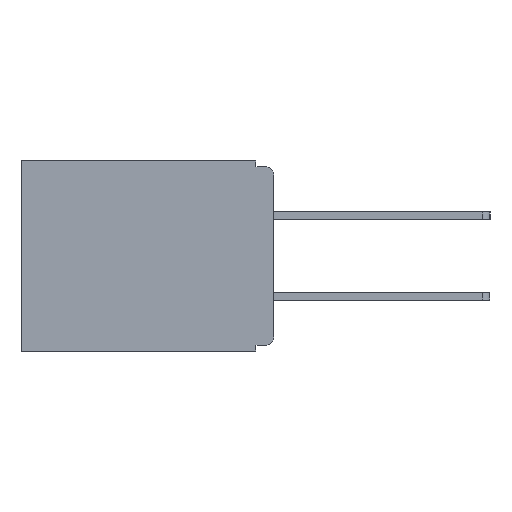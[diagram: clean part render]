
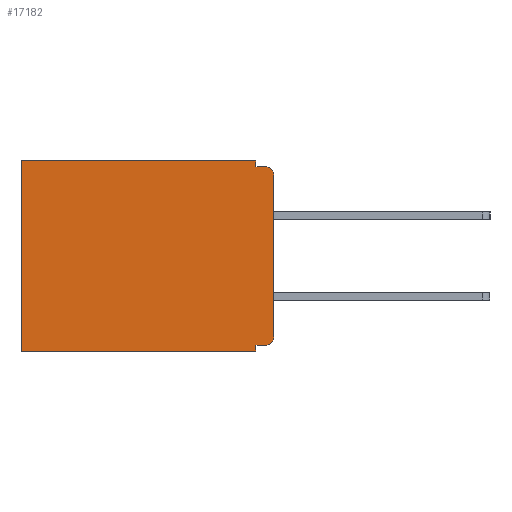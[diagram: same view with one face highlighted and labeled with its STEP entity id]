
A CAD part, left-side view. The second image highlights one B-rep face of the part: STEP entity #17182.
In plain terms, the highlighted planar face has unit normal (-1, 0, 0).
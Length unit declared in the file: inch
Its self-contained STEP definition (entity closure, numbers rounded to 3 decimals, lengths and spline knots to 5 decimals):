
#286 = DIRECTION ( 'NONE',  ( 0., 0., -1. ) ) ;
#375 = ORIENTED_EDGE ( 'NONE', *, *, #14179, .F. ) ;
#651 = LINE ( 'NONE', #19737, #20447 ) ;
#837 = EDGE_CURVE ( 'NONE', #881, #17646, #8882, .T. ) ;
#881 = VERTEX_POINT ( 'NONE', #23216 ) ;
#1035 = LINE ( 'NONE', #2843, #15155 ) ;
#1166 = ORIENTED_EDGE ( 'NONE', *, *, #12074, .T. ) ;
#1326 = VERTEX_POINT ( 'NONE', #3470 ) ;
#2004 = AXIS2_PLACEMENT_3D ( 'NONE', #9203, #22549, #11126 ) ;
#2218 = ORIENTED_EDGE ( 'NONE', *, *, #837, .F. ) ;
#2843 = CARTESIAN_POINT ( 'NONE',  ( 0.3, 0., -0.01 ) ) ;
#3128 = CARTESIAN_POINT ( 'NONE',  ( 0.3, 0.031, 0. ) ) ;
#3470 = CARTESIAN_POINT ( 'NONE',  ( 0.3, 0.031, 0. ) ) ;
#3496 = DIRECTION ( 'NONE',  ( 0., 1., 0. ) ) ;
#5076 = DIRECTION ( 'NONE',  ( 0., 0., -1. ) ) ;
#5280 = CARTESIAN_POINT ( 'NONE',  ( 0.3, 0.015, -0.01 ) ) ;
#5361 = DIRECTION ( 'NONE',  ( 1., 0., 0. ) ) ;
#5703 = EDGE_CURVE ( 'NONE', #19133, #17646, #16681, .T. ) ;
#5920 = VERTEX_POINT ( 'NONE', #5280 ) ;
#6975 = VERTEX_POINT ( 'NONE', #13153 ) ;
#7136 = EDGE_LOOP ( 'NONE', ( #2218, #1166, #375, #15048, #14699, #13847, #13239, #12984, #12619, #12115 ) ) ;
#7376 = VERTEX_POINT ( 'NONE', #16250 ) ;
#8443 = CARTESIAN_POINT ( 'NONE',  ( 0.3, 0.437, 0. ) ) ;
#8515 = DIRECTION ( 'NONE',  ( 0., -1., 0. ) ) ;
#8859 = CARTESIAN_POINT ( 'NONE',  ( 0.3, 0.031, -0.33 ) ) ;
#8880 = LINE ( 'NONE', #8859, #22339 ) ;
#8882 = LINE ( 'NONE', #13978, #19072 ) ;
#9203 = CARTESIAN_POINT ( 'NONE',  ( 0.3, 0.015, -0.025 ) ) ;
#9400 = CARTESIAN_POINT ( 'NONE',  ( 0.3, 0.437, -0.33 ) ) ;
#9470 = AXIS2_PLACEMENT_3D ( 'NONE', #19994, #11107, #286 ) ;
#9677 = EDGE_CURVE ( 'NONE', #13610, #7376, #20761, .T. ) ;
#9882 = CARTESIAN_POINT ( 'NONE',  ( 0.3, 0., -0.32 ) ) ;
#10412 = VECTOR ( 'NONE', #5076, 39.37008 ) ;
#10506 = EDGE_CURVE ( 'NONE', #10758, #7376, #651, .T. ) ;
#10758 = VERTEX_POINT ( 'NONE', #12755 ) ;
#11087 = CARTESIAN_POINT ( 'NONE',  ( 0.3, 0., 0. ) ) ;
#11107 = DIRECTION ( 'NONE',  ( -1., 0., 0. ) ) ;
#11126 = DIRECTION ( 'NONE',  ( 0., 0., -1. ) ) ;
#11375 = FACE_OUTER_BOUND ( 'NONE', #7136, .T. ) ;
#11613 = CARTESIAN_POINT ( 'NONE',  ( 0.3, 0.031, -0.01 ) ) ;
#12074 = EDGE_CURVE ( 'NONE', #881, #5920, #12242, .T. ) ;
#12115 = ORIENTED_EDGE ( 'NONE', *, *, #5703, .T. ) ;
#12242 = CIRCLE ( 'NONE', #2004, 0.015 ) ;
#12579 = VECTOR ( 'NONE', #3496, 39.37008 ) ;
#12619 = ORIENTED_EDGE ( 'NONE', *, *, #22333, .F. ) ;
#12755 = CARTESIAN_POINT ( 'NONE',  ( 0.3, 0.031, -0.33 ) ) ;
#12984 = ORIENTED_EDGE ( 'NONE', *, *, #18687, .F. ) ;
#13153 = CARTESIAN_POINT ( 'NONE',  ( 0.3, 0.031, -0.32 ) ) ;
#13239 = ORIENTED_EDGE ( 'NONE', *, *, #10506, .F. ) ;
#13610 = VERTEX_POINT ( 'NONE', #8443 ) ;
#13847 = ORIENTED_EDGE ( 'NONE', *, *, #9677, .T. ) ;
#13978 = CARTESIAN_POINT ( 'NONE',  ( 0.3, 0., -0.33 ) ) ;
#14087 = VECTOR ( 'NONE', #21343, 39.37008 ) ;
#14179 = EDGE_CURVE ( 'NONE', #22879, #5920, #1035, .T. ) ;
#14683 = LINE ( 'NONE', #9882, #14087 ) ;
#14699 = ORIENTED_EDGE ( 'NONE', *, *, #21457, .T. ) ;
#14764 = CARTESIAN_POINT ( 'NONE',  ( 0.3, 0., -0.305 ) ) ;
#15048 = ORIENTED_EDGE ( 'NONE', *, *, #23754, .F. ) ;
#15078 = VECTOR ( 'NONE', #24606, 39.37008 ) ;
#15155 = VECTOR ( 'NONE', #8515, 39.37008 ) ;
#15517 = LINE ( 'NONE', #3128, #10412 ) ;
#16250 = CARTESIAN_POINT ( 'NONE',  ( 0.3, 0.437, -0.33 ) ) ;
#16681 = CIRCLE ( 'NONE', #9470, 0.015 ) ;
#16805 = CARTESIAN_POINT ( 'NONE',  ( 0.3, 0., -0.33 ) ) ;
#17182 = ADVANCED_FACE ( 'NONE', ( #11375 ), #20560, .F. ) ;
#17646 = VERTEX_POINT ( 'NONE', #14764 ) ;
#17699 = LINE ( 'NONE', #11087, #12579 ) ;
#18687 = EDGE_CURVE ( 'NONE', #6975, #10758, #8880, .T. ) ;
#18713 = DIRECTION ( 'NONE',  ( 0., 0., -1. ) ) ;
#18759 = AXIS2_PLACEMENT_3D ( 'NONE', #16805, #5361, #18713 ) ;
#19072 = VECTOR ( 'NONE', #19273, 39.37008 ) ;
#19133 = VERTEX_POINT ( 'NONE', #23594 ) ;
#19273 = DIRECTION ( 'NONE',  ( 0., 0., -1. ) ) ;
#19737 = CARTESIAN_POINT ( 'NONE',  ( 0.3, 0., -0.33 ) ) ;
#19994 = CARTESIAN_POINT ( 'NONE',  ( 0.3, 0.015, -0.305 ) ) ;
#20447 = VECTOR ( 'NONE', #23528, 39.37008 ) ;
#20560 = PLANE ( 'NONE',  #18759 ) ;
#20761 = LINE ( 'NONE', #9400, #15078 ) ;
#21343 = DIRECTION ( 'NONE',  ( 0., 1., 0. ) ) ;
#21457 = EDGE_CURVE ( 'NONE', #1326, #13610, #17699, .T. ) ;
#22333 = EDGE_CURVE ( 'NONE', #19133, #6975, #14683, .T. ) ;
#22339 = VECTOR ( 'NONE', #24092, 39.37008 ) ;
#22549 = DIRECTION ( 'NONE',  ( -1., 0., 0. ) ) ;
#22879 = VERTEX_POINT ( 'NONE', #11613 ) ;
#23216 = CARTESIAN_POINT ( 'NONE',  ( 0.3, 0., -0.025 ) ) ;
#23528 = DIRECTION ( 'NONE',  ( 0., 1., 0. ) ) ;
#23594 = CARTESIAN_POINT ( 'NONE',  ( 0.3, 0.015, -0.32 ) ) ;
#23754 = EDGE_CURVE ( 'NONE', #1326, #22879, #15517, .T. ) ;
#24092 = DIRECTION ( 'NONE',  ( 0., 0., -1. ) ) ;
#24606 = DIRECTION ( 'NONE',  ( 0., 0., -1. ) ) ;
